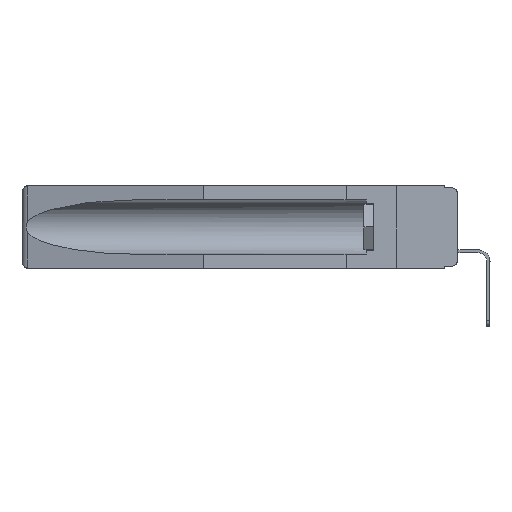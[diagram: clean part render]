
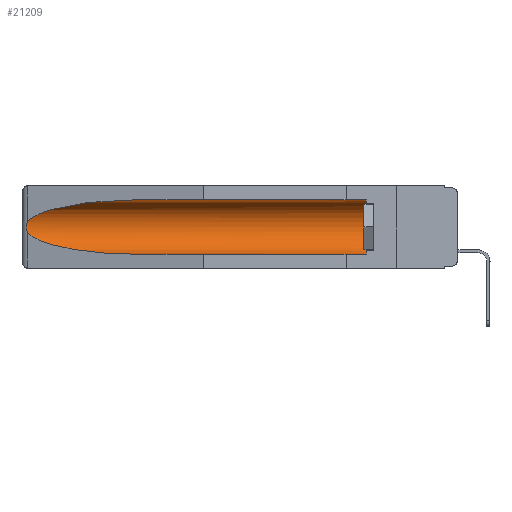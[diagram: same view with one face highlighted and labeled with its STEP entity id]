
A CAD part, left-side view. The second image highlights one B-rep face of the part: STEP entity #21209.
In plain terms, the highlighted cylindrical face has radius 2.857 mm (diameter 5.715 mm), a partial arc.
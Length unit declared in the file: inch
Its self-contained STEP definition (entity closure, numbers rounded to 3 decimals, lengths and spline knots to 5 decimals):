
#641 = EDGE_CURVE ( 'NONE', #20508, #1546, #20506, .T. ) ;
#646 = CARTESIAN_POINT ( 'NONE',  ( 0.25451, 1.48313, -0.24835 ) ) ;
#1055 = ORIENTED_EDGE ( 'NONE', *, *, #2913, .T. ) ;
#1371 = CARTESIAN_POINT ( 'NONE',  ( 0.21114, 1.30732, -0.059 ) ) ;
#1546 = VERTEX_POINT ( 'NONE', #8616 ) ;
#1582 = DIRECTION ( 'NONE',  ( 0., 0., 1. ) ) ;
#1595 = AXIS2_PLACEMENT_3D ( 'NONE', #13895, #14058, #4857 ) ;
#2128 = CARTESIAN_POINT ( 'NONE',  ( 0.26654, 1.53092, -0.15636 ) ) ;
#2670 = ORIENTED_EDGE ( 'NONE', *, *, #641, .F. ) ;
#2913 = EDGE_CURVE ( 'NONE', #8846, #23570, #4352, .T. ) ;
#3211 = ORIENTED_EDGE ( 'NONE', *, *, #15222, .T. ) ;
#3858 = EDGE_LOOP ( 'NONE', ( #17680, #1055, #8990, #2670, #9324, #3211 ) ) ;
#4234 = CARTESIAN_POINT ( 'NONE',  ( 0.21114, 1.30732, -0.284 ) ) ;
#4352 = B_SPLINE_CURVE_WITH_KNOTS ( 'NONE', 3,
 ( #14950, #16791, #2128, #16879, #18723, #7707, #20559, #13352, #6338, #19052 ),
 .UNSPECIFIED., .F., .F.,
 ( 4, 2, 2, 2, 4 ),
 ( 0., 0.00029, 0.00058, 0.00087, 0.00117 ),
 .UNSPECIFIED. ) ;
#4857 = DIRECTION ( 'NONE',  ( 0., 0., 1. ) ) ;
#6338 = CARTESIAN_POINT ( 'NONE',  ( 0.26597, 1.5296, -0.19026 ) ) ;
#6394 = CARTESIAN_POINT ( 'NONE',  ( 0.155, 1.07973, -0.284 ) ) ;
#7234 = CARTESIAN_POINT ( 'NONE',  ( 0.155, -0.30754, -0.284 ) ) ;
#7707 = CARTESIAN_POINT ( 'NONE',  ( 0.2675, 1.53308, -0.17534 ) ) ;
#8616 = CARTESIAN_POINT ( 'NONE',  ( 0.155, 1.07973, -0.284 ) ) ;
#8817 = CARTESIAN_POINT ( 'NONE',  ( 0.25451, 1.48313, -0.09465 ) ) ;
#8846 = VERTEX_POINT ( 'NONE', #16897 ) ;
#8990 = ORIENTED_EDGE ( 'NONE', *, *, #20996, .T. ) ;
#9324 = ORIENTED_EDGE ( 'NONE', *, *, #9473, .T. ) ;
#9398 = DIRECTION ( 'NONE',  ( 0., 1., 0. ) ) ;
#9473 = EDGE_CURVE ( 'NONE', #20508, #22975, #17872, .T. ) ;
#10564 = VERTEX_POINT ( 'NONE', #13697 ) ;
#10751 = EDGE_CURVE ( 'NONE', #10564, #8846, #18207, .T. ) ;
#10782 = DIRECTION ( 'NONE',  ( 0., -1., 0. ) ) ;
#12296 = CARTESIAN_POINT ( 'NONE',  ( 0.26537, 1.52718, -0.19328 ) ) ;
#13352 = CARTESIAN_POINT ( 'NONE',  ( 0.26655, 1.53094, -0.18657 ) ) ;
#13697 = CARTESIAN_POINT ( 'NONE',  ( 0.155, 1.07973, -0.059 ) ) ;
#13895 = CARTESIAN_POINT ( 'NONE',  ( 0.155, -0.30754, -0.1715 ) ) ;
#13910 = CYLINDRICAL_SURFACE ( 'NONE', #1595, 0.1125 ) ;
#14013 = CARTESIAN_POINT ( 'NONE',  ( 0.155, 0.126, -0.284 ) ) ;
#14058 = DIRECTION ( 'NONE',  ( 0., 1., 0. ) ) ;
#14133 = CARTESIAN_POINT ( 'NONE',  ( 0.155, 0.126, -0.059 ) ) ;
#14367 = CARTESIAN_POINT ( 'NONE',  ( 0.26537, 1.52718, -0.14972 ) ) ;
#14950 = CARTESIAN_POINT ( 'NONE',  ( 0.26537, 1.52718, -0.14972 ) ) ;
#15222 = EDGE_CURVE ( 'NONE', #22975, #10564, #16111, .T. ) ;
#15346 = CARTESIAN_POINT ( 'NONE',  ( 0.26537, 1.52718, -0.19328 ) ) ;
#15636 = AXIS2_PLACEMENT_3D ( 'NONE', #16819, #10782, #1582 ) ;
#16111 = LINE ( 'NONE', #21704, #20122 ) ;
#16791 = CARTESIAN_POINT ( 'NONE',  ( 0.26597, 1.52961, -0.15275 ) ) ;
#16819 = CARTESIAN_POINT ( 'NONE',  ( 0.155, 0.126, -0.1715 ) ) ;
#16879 = CARTESIAN_POINT ( 'NONE',  ( 0.2673, 1.5327, -0.16383 ) ) ;
#16897 = CARTESIAN_POINT ( 'NONE',  ( 0.26537, 1.52718, -0.14972 ) ) ;
#17469 =( BOUNDED_CURVE ( )  B_SPLINE_CURVE ( 3, ( #15346, #646, #4234, #6394 ),
 .UNSPECIFIED., .F., .F. ) 
 B_SPLINE_CURVE_WITH_KNOTS ( ( 4, 4 ),
 ( 0.1948, 1.5708 ),
 .UNSPECIFIED. ) 
 CURVE ( )  GEOMETRIC_REPRESENTATION_ITEM ( )  RATIONAL_B_SPLINE_CURVE ( ( 1., 0.848, 0.848, 1. ) ) 
 REPRESENTATION_ITEM ( '' )  );
#17680 = ORIENTED_EDGE ( 'NONE', *, *, #10751, .T. ) ;
#17872 = CIRCLE ( 'NONE', #15636, 0.1125 ) ;
#18196 = FACE_OUTER_BOUND ( 'NONE', #3858, .T. ) ;
#18207 =( BOUNDED_CURVE ( )  B_SPLINE_CURVE ( 3, ( #23431, #1371, #8817, #14367 ),
 .UNSPECIFIED., .F., .F. ) 
 B_SPLINE_CURVE_WITH_KNOTS ( ( 4, 4 ),
 ( 4.71239, 6.08839 ),
 .UNSPECIFIED. ) 
 CURVE ( )  GEOMETRIC_REPRESENTATION_ITEM ( )  RATIONAL_B_SPLINE_CURVE ( ( 1., 0.848, 0.848, 1. ) ) 
 REPRESENTATION_ITEM ( '' )  );
#18723 = CARTESIAN_POINT ( 'NONE',  ( 0.2675, 1.53308, -0.16763 ) ) ;
#19052 = CARTESIAN_POINT ( 'NONE',  ( 0.26537, 1.52718, -0.19328 ) ) ;
#20122 = VECTOR ( 'NONE', #9398, 39.37008 ) ;
#20506 = LINE ( 'NONE', #7234, #23101 ) ;
#20508 = VERTEX_POINT ( 'NONE', #14013 ) ;
#20559 = CARTESIAN_POINT ( 'NONE',  ( 0.2673, 1.53269, -0.17917 ) ) ;
#20996 = EDGE_CURVE ( 'NONE', #23570, #1546, #17469, .T. ) ;
#21209 = ADVANCED_FACE ( 'NONE', ( #18196 ), #13910, .F. ) ;
#21704 = CARTESIAN_POINT ( 'NONE',  ( 0.155, -0.30754, -0.059 ) ) ;
#22975 = VERTEX_POINT ( 'NONE', #14133 ) ;
#23101 = VECTOR ( 'NONE', #23710, 39.37008 ) ;
#23431 = CARTESIAN_POINT ( 'NONE',  ( 0.155, 1.07973, -0.059 ) ) ;
#23570 = VERTEX_POINT ( 'NONE', #12296 ) ;
#23710 = DIRECTION ( 'NONE',  ( 0., 1., 0. ) ) ;
